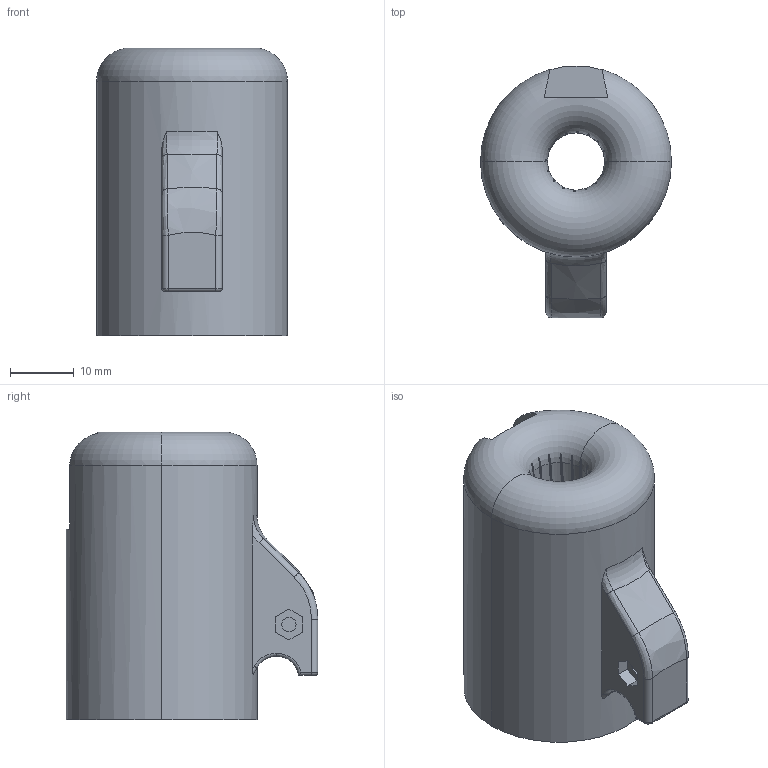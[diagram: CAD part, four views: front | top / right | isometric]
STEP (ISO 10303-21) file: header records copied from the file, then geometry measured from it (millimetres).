
FILE_DESCRIPTION (( 'STEP AP214' ), '1' );
FILE_NAME ('Barrel_.380_ACP.step', '2013-11-06T14:30:41', ( 'elpi' ), ( '' ), 'SwSTEP 2.0', 'SolidWorks 2013', '' );
FILE_SCHEMA (( 'AUTOMOTIVE_DESIGN' ));
Length unit declared in the file: millimetre
Products named in the file (1): Barrel_.380_ACP
Bounding box: 30 x 39.54 x 45.25 mm (x, y, z)
Volume: 29004.6 mm3; surface area: 7414.6 mm2
Topology: 1 solids, 1 shells, 337 faces, 814 edges, 451 vertices
Faces by surface type: bspline 247, cylinder 35, torus 27, plane 25, cone 3
Entity records: 19018 total; most frequent: CARTESIAN_POINT 13087, ORIENTED_EDGE 1564, EDGE_CURVE 782, DIRECTION 777, VERTEX_POINT 451, B_SPLINE_CURVE_WITH_KNOTS 449, AXIS2_PLACEMENT_3D 353, EDGE_LOOP 343
